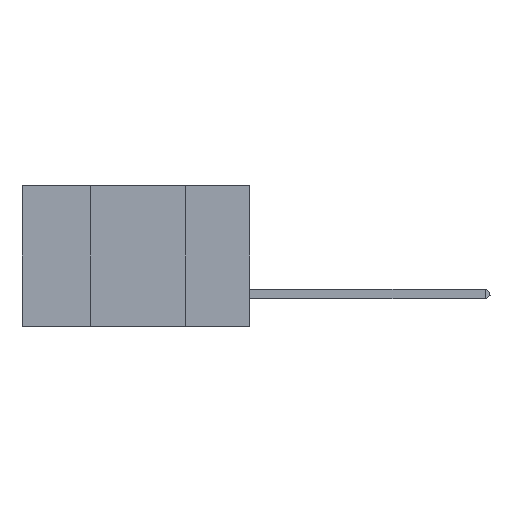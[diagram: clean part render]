
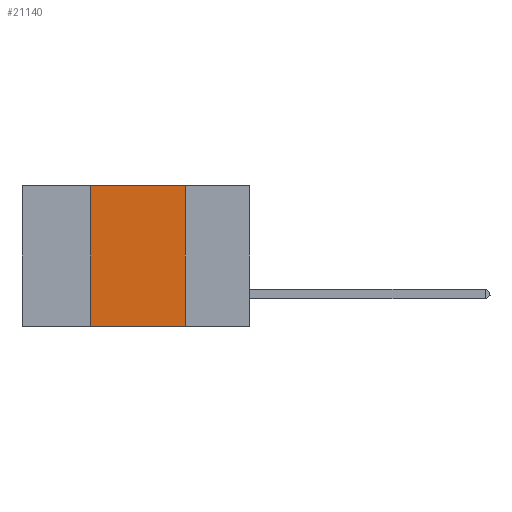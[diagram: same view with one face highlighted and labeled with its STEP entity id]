
A CAD part, left-side view. The second image highlights one B-rep face of the part: STEP entity #21140.
In plain terms, the highlighted planar face has unit normal (-1, 0, 0).
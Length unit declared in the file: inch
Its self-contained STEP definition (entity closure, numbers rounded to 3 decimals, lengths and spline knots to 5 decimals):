
#65 = VECTOR ( 'NONE', #4872, 39.37008 ) ;
#1013 = EDGE_LOOP ( 'NONE', ( #16845, #16526, #1632, #14829 ) ) ;
#1632 = ORIENTED_EDGE ( 'NONE', *, *, #16782, .F. ) ;
#1726 = CARTESIAN_POINT ( 'NONE',  ( 0., 0.42, -0.37 ) ) ;
#2507 = LINE ( 'NONE', #18429, #21452 ) ;
#3976 = VERTEX_POINT ( 'NONE', #1726 ) ;
#4441 = VERTEX_POINT ( 'NONE', #17988 ) ;
#4620 = CARTESIAN_POINT ( 'NONE',  ( 0., 0.42, 0. ) ) ;
#4721 = LINE ( 'NONE', #8285, #65 ) ;
#4872 = DIRECTION ( 'NONE',  ( 0., -1., 0. ) ) ;
#5097 = VECTOR ( 'NONE', #15059, 39.37008 ) ;
#5224 = AXIS2_PLACEMENT_3D ( 'NONE', #17564, #20704, #19154 ) ;
#5492 = EDGE_CURVE ( 'NONE', #4441, #6334, #2507, .T. ) ;
#5742 = DIRECTION ( 'NONE',  ( 0., 0., -1. ) ) ;
#6334 = VERTEX_POINT ( 'NONE', #16030 ) ;
#8285 = CARTESIAN_POINT ( 'NONE',  ( 0., 0.6, -0.37 ) ) ;
#8409 = LINE ( 'NONE', #9940, #18666 ) ;
#8595 = PLANE ( 'NONE',  #5224 ) ;
#9804 = FACE_OUTER_BOUND ( 'NONE', #1013, .T. ) ;
#9940 = CARTESIAN_POINT ( 'NONE',  ( 0., 0.6, 0. ) ) ;
#12629 = EDGE_CURVE ( 'NONE', #14894, #4441, #8409, .T. ) ;
#14131 = CARTESIAN_POINT ( 'NONE',  ( 0., 0.42, 0. ) ) ;
#14829 = ORIENTED_EDGE ( 'NONE', *, *, #15915, .T. ) ;
#14894 = VERTEX_POINT ( 'NONE', #14131 ) ;
#14994 = DIRECTION ( 'NONE',  ( 0., -1., 0. ) ) ;
#15059 = DIRECTION ( 'NONE',  ( 0., 0., 1. ) ) ;
#15915 = EDGE_CURVE ( 'NONE', #3976, #6334, #4721, .T. ) ;
#16030 = CARTESIAN_POINT ( 'NONE',  ( 0., 0.17, -0.37 ) ) ;
#16526 = ORIENTED_EDGE ( 'NONE', *, *, #12629, .F. ) ;
#16782 = EDGE_CURVE ( 'NONE', #3976, #14894, #19123, .T. ) ;
#16845 = ORIENTED_EDGE ( 'NONE', *, *, #5492, .F. ) ;
#17564 = CARTESIAN_POINT ( 'NONE',  ( 0., 0.6, 0. ) ) ;
#17988 = CARTESIAN_POINT ( 'NONE',  ( 0., 0.17, 0. ) ) ;
#18429 = CARTESIAN_POINT ( 'NONE',  ( 0., 0.17, 0. ) ) ;
#18666 = VECTOR ( 'NONE', #14994, 39.37008 ) ;
#19123 = LINE ( 'NONE', #4620, #5097 ) ;
#19154 = DIRECTION ( 'NONE',  ( 0., 0., -1. ) ) ;
#20704 = DIRECTION ( 'NONE',  ( 1., 0., 0. ) ) ;
#21140 = ADVANCED_FACE ( 'NONE', ( #9804 ), #8595, .F. ) ;
#21452 = VECTOR ( 'NONE', #5742, 39.37008 ) ;
